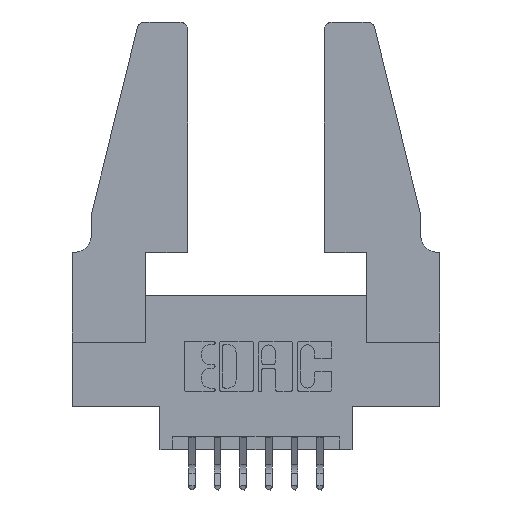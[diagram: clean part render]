
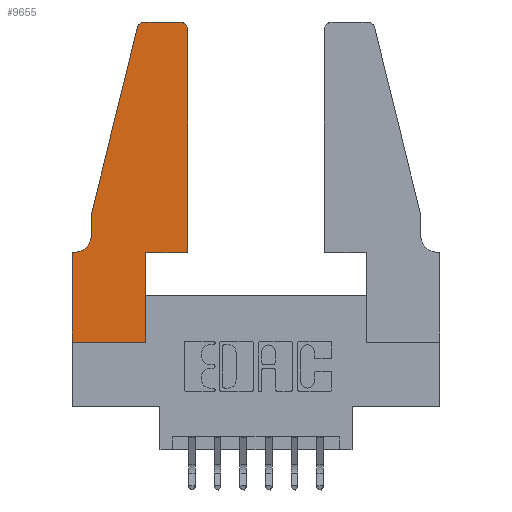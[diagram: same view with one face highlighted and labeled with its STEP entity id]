
A CAD part, top view. The second image highlights one B-rep face of the part: STEP entity #9655.
In plain terms, the highlighted planar face has unit normal (0, 0, 1).
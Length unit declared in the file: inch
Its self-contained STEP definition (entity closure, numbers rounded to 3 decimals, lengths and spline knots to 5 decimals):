
#83 = EDGE_LOOP ( 'NONE', ( #413, #3440, #9300, #3647, #6339, #3660, #7220, #4883, #921, #11898, #2227, #4652 ) ) ;
#97 = CARTESIAN_POINT ( 'NONE',  ( 0.0755, 0.42, 0.37 ) ) ;
#170 = VERTEX_POINT ( 'NONE', #4453 ) ;
#376 = CARTESIAN_POINT ( 'NONE',  ( 0.4505, 0.35, 0.37 ) ) ;
#413 = ORIENTED_EDGE ( 'NONE', *, *, #12009, .T. ) ;
#598 = EDGE_CURVE ( 'NONE', #8351, #2499, #10611, .T. ) ;
#921 = ORIENTED_EDGE ( 'NONE', *, *, #8058, .T. ) ;
#966 = VERTEX_POINT ( 'NONE', #8752 ) ;
#1014 = VERTEX_POINT ( 'NONE', #1078 ) ;
#1078 = CARTESIAN_POINT ( 'NONE',  ( 0., 0., 0.37 ) ) ;
#1093 = CARTESIAN_POINT ( 'NONE',  ( 0.2605, 1.25, 0.37 ) ) ;
#1277 = FACE_OUTER_BOUND ( 'NONE', #83, .T. ) ;
#1346 = VERTEX_POINT ( 'NONE', #3250 ) ;
#1601 = VERTEX_POINT ( 'NONE', #8357 ) ;
#2001 = LINE ( 'NONE', #1093, #11251 ) ;
#2100 = AXIS2_PLACEMENT_3D ( 'NONE', #4443, #10784, #5407 ) ;
#2172 = EDGE_CURVE ( 'NONE', #966, #8187, #11944, .T. ) ;
#2227 = ORIENTED_EDGE ( 'NONE', *, *, #10679, .T. ) ;
#2346 = CARTESIAN_POINT ( 'NONE',  ( 0.4505, 0.35, 0.37 ) ) ;
#2374 = CARTESIAN_POINT ( 'NONE',  ( 0., 0., 0.37 ) ) ;
#2437 = VERTEX_POINT ( 'NONE', #12042 ) ;
#2499 = VERTEX_POINT ( 'NONE', #97 ) ;
#2646 = LINE ( 'NONE', #6202, #4357 ) ;
#2661 = CARTESIAN_POINT ( 'NONE',  ( 0., 0.35, 0.37 ) ) ;
#2752 = CARTESIAN_POINT ( 'NONE',  ( 0.0055, 0.42, 0.37 ) ) ;
#2794 = VECTOR ( 'NONE', #4590, 39.37008 ) ;
#3033 = CARTESIAN_POINT ( 'NONE',  ( 0.2865, 0.35, 0.37 ) ) ;
#3250 = CARTESIAN_POINT ( 'NONE',  ( 0.25487, 1.22718, 0.37 ) ) ;
#3253 = LINE ( 'NONE', #2374, #10055 ) ;
#3267 = VECTOR ( 'NONE', #6568, 39.37008 ) ;
#3271 = CARTESIAN_POINT ( 'NONE',  ( 0.4505, 1.22, 0.37 ) ) ;
#3315 = VERTEX_POINT ( 'NONE', #8685 ) ;
#3440 = ORIENTED_EDGE ( 'NONE', *, *, #4464, .T. ) ;
#3459 = CARTESIAN_POINT ( 'NONE',  ( 0.0755, 0.5, 0.37 ) ) ;
#3647 = ORIENTED_EDGE ( 'NONE', *, *, #598, .T. ) ;
#3651 = DIRECTION ( 'NONE',  ( 1., 0., 0. ) ) ;
#3660 = ORIENTED_EDGE ( 'NONE', *, *, #10696, .T. ) ;
#3728 = DIRECTION ( 'NONE',  ( -1., 0., 0. ) ) ;
#3841 = LINE ( 'NONE', #5873, #8537 ) ;
#4332 = DIRECTION ( 'NONE',  ( 0., 1., 0. ) ) ;
#4357 = VECTOR ( 'NONE', #10688, 39.37008 ) ;
#4443 = CARTESIAN_POINT ( 'NONE',  ( 0.4205, 1.22, 0.37 ) ) ;
#4453 = CARTESIAN_POINT ( 'NONE',  ( 0.2865, 0., 0.37 ) ) ;
#4464 = EDGE_CURVE ( 'NONE', #2437, #1346, #5733, .T. ) ;
#4590 = DIRECTION ( 'NONE',  ( -0.239, -0.971, 0. ) ) ;
#4610 = VERTEX_POINT ( 'NONE', #8734 ) ;
#4652 = ORIENTED_EDGE ( 'NONE', *, *, #11592, .T. ) ;
#4758 = VERTEX_POINT ( 'NONE', #3271 ) ;
#4883 = ORIENTED_EDGE ( 'NONE', *, *, #7017, .T. ) ;
#5131 = AXIS2_PLACEMENT_3D ( 'NONE', #2661, #9220, #3651 ) ;
#5183 = CARTESIAN_POINT ( 'NONE',  ( 0.4505, 0.35, 0.37 ) ) ;
#5407 = DIRECTION ( 'NONE',  ( 1., 0., 0. ) ) ;
#5733 = CIRCLE ( 'NONE', #6440, 0.03 ) ;
#5804 = CARTESIAN_POINT ( 'NONE',  ( 0.284, 1.22, 0.37 ) ) ;
#5851 = CIRCLE ( 'NONE', #6391, 0.07 ) ;
#5873 = CARTESIAN_POINT ( 'NONE',  ( 0., 0., 0.37 ) ) ;
#5943 = DIRECTION ( 'NONE',  ( 0., 1., 0. ) ) ;
#5952 = DIRECTION ( 'NONE',  ( -1., 0., 0. ) ) ;
#6202 = CARTESIAN_POINT ( 'NONE',  ( 0.0755, 0.35, 0.37 ) ) ;
#6248 = CARTESIAN_POINT ( 'NONE',  ( 0.0755, 0.5, 0.37 ) ) ;
#6339 = ORIENTED_EDGE ( 'NONE', *, *, #9687, .T. ) ;
#6391 = AXIS2_PLACEMENT_3D ( 'NONE', #2752, #9297, #3728 ) ;
#6440 = AXIS2_PLACEMENT_3D ( 'NONE', #5804, #12076, #6757 ) ;
#6568 = DIRECTION ( 'NONE',  ( 0., -1., 0. ) ) ;
#6757 = DIRECTION ( 'NONE',  ( 1., 0., 0. ) ) ;
#7017 = EDGE_CURVE ( 'NONE', #1014, #170, #3253, .T. ) ;
#7220 = ORIENTED_EDGE ( 'NONE', *, *, #7440, .T. ) ;
#7440 = EDGE_CURVE ( 'NONE', #1601, #1014, #3841, .T. ) ;
#7764 = DIRECTION ( 'NONE',  ( 0., -1., 0. ) ) ;
#8058 = EDGE_CURVE ( 'NONE', #170, #966, #9201, .T. ) ;
#8187 = VERTEX_POINT ( 'NONE', #5183 ) ;
#8351 = VERTEX_POINT ( 'NONE', #3459 ) ;
#8357 = CARTESIAN_POINT ( 'NONE',  ( 0., 0.35, 0.37 ) ) ;
#8361 = PLANE ( 'NONE',  #5131 ) ;
#8537 = VECTOR ( 'NONE', #7764, 39.37008 ) ;
#8684 = CIRCLE ( 'NONE', #2100, 0.03 ) ;
#8685 = CARTESIAN_POINT ( 'NONE',  ( 0.0055, 0.35, 0.37 ) ) ;
#8734 = CARTESIAN_POINT ( 'NONE',  ( 0.4205, 1.25, 0.37 ) ) ;
#8752 = CARTESIAN_POINT ( 'NONE',  ( 0.2865, 0.35, 0.37 ) ) ;
#9201 = LINE ( 'NONE', #3033, #11525 ) ;
#9220 = DIRECTION ( 'NONE',  ( 0., 0., 1. ) ) ;
#9297 = DIRECTION ( 'NONE',  ( 0., 0., -1. ) ) ;
#9300 = ORIENTED_EDGE ( 'NONE', *, *, #10844, .T. ) ;
#9655 = ADVANCED_FACE ( 'NONE', ( #1277 ), #8361, .T. ) ;
#9687 = EDGE_CURVE ( 'NONE', #2499, #3315, #5851, .T. ) ;
#9929 = LINE ( 'NONE', #10910, #2794 ) ;
#10055 = VECTOR ( 'NONE', #11598, 39.37008 ) ;
#10611 = LINE ( 'NONE', #6248, #3267 ) ;
#10679 = EDGE_CURVE ( 'NONE', #8187, #4758, #11868, .T. ) ;
#10688 = DIRECTION ( 'NONE',  ( -1., 0., 0. ) ) ;
#10696 = EDGE_CURVE ( 'NONE', #3315, #1601, #2646, .T. ) ;
#10784 = DIRECTION ( 'NONE',  ( 0., 0., 1. ) ) ;
#10844 = EDGE_CURVE ( 'NONE', #1346, #8351, #9929, .T. ) ;
#10910 = CARTESIAN_POINT ( 'NONE',  ( 0.0755, 0.5, 0.37 ) ) ;
#11251 = VECTOR ( 'NONE', #5952, 39.37008 ) ;
#11373 = VECTOR ( 'NONE', #11689, 39.37008 ) ;
#11525 = VECTOR ( 'NONE', #5943, 39.37008 ) ;
#11569 = VECTOR ( 'NONE', #4332, 39.37008 ) ;
#11592 = EDGE_CURVE ( 'NONE', #4758, #4610, #8684, .T. ) ;
#11598 = DIRECTION ( 'NONE',  ( 1., 0., 0. ) ) ;
#11689 = DIRECTION ( 'NONE',  ( 1., 0., 0. ) ) ;
#11868 = LINE ( 'NONE', #2346, #11569 ) ;
#11898 = ORIENTED_EDGE ( 'NONE', *, *, #2172, .T. ) ;
#11944 = LINE ( 'NONE', #376, #11373 ) ;
#12009 = EDGE_CURVE ( 'NONE', #4610, #2437, #2001, .T. ) ;
#12042 = CARTESIAN_POINT ( 'NONE',  ( 0.284, 1.25, 0.37 ) ) ;
#12076 = DIRECTION ( 'NONE',  ( 0., 0., 1. ) ) ;
